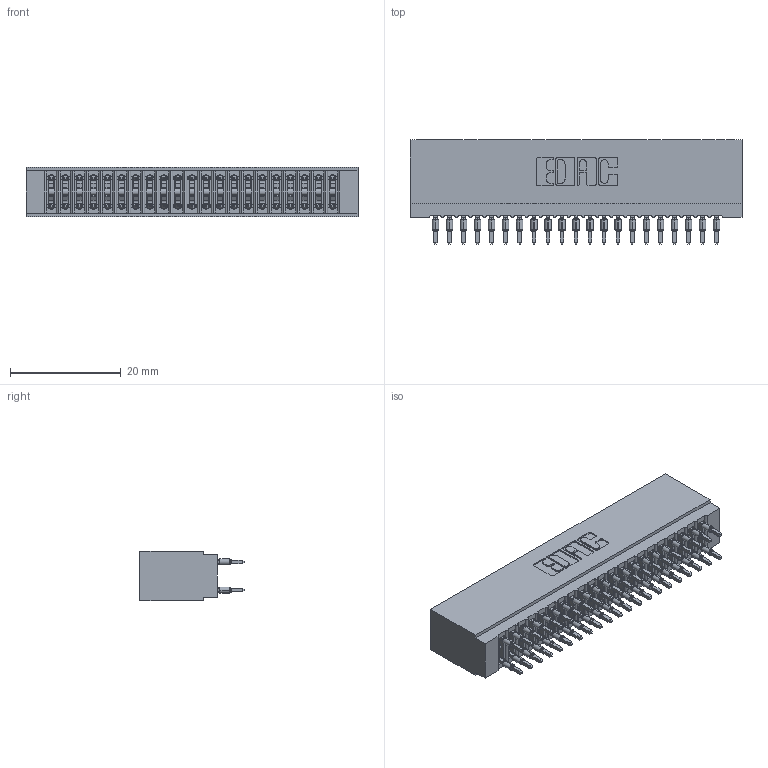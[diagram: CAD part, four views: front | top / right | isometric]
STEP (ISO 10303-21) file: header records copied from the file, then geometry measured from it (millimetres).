
FILE_DESCRIPTION (( 'STEP AP203' ), '1' );
FILE_NAME ('725-042-560-201.STEP', '2026-02-24T17:35:20', ( '' ), ( '' ), 'SwSTEP 2.0', 'SolidWorks 2023', '' );
FILE_SCHEMA (( 'CONFIG_CONTROL_DESIGN' ));
Length unit declared in the file: millimetre
Products named in the file (3): 725-042-560-201; 745-292-001_560; 725 Part_Insulator Option - 01
Assembly tree (43 placements, depth 2):
  725-042-560-201
    725 Part_Insulator Option - 01
    745-292-001_560  x42
Bounding box: 59.94 x 18.8 x 8.89 mm (x, y, z)
Volume: 5014.6 mm3; surface area: 10804.5 mm2
Topology: 43 solids, 43 shells, 4232 faces, 11573 edges, 7350 vertices
Faces by surface type: plane 2197, cylinder 943, bspline 840, torus 252
Entity records: 38508 total; most frequent: CARTESIAN_POINT 7189, ORIENTED_EDGE 6582, DIRECTION 5775, EDGE_CURVE 3291, LINE 2975, VECTOR 2975, VERTEX_POINT 2102, AXIS2_PLACEMENT_3D 1400
